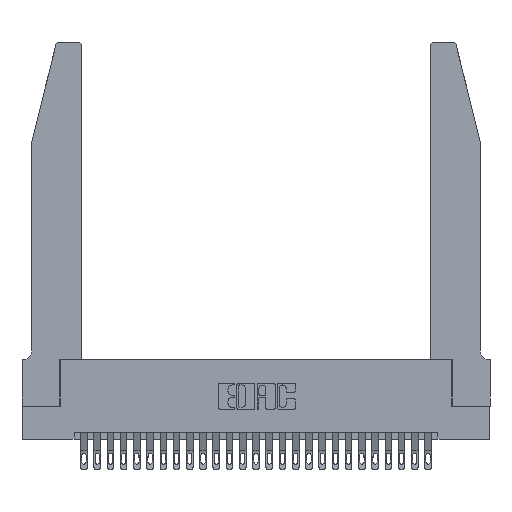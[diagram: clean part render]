
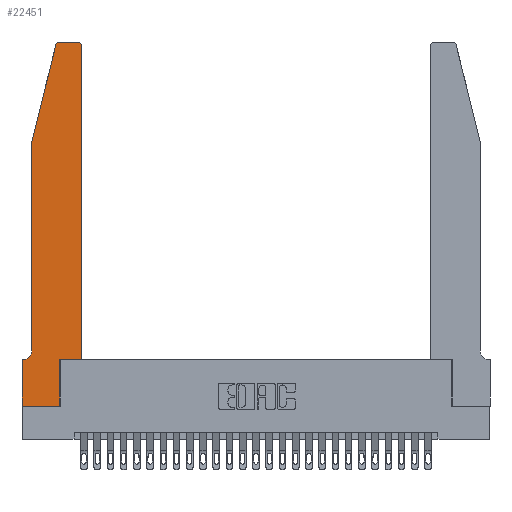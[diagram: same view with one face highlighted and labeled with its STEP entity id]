
A CAD part, top view. The second image highlights one B-rep face of the part: STEP entity #22451.
In plain terms, the highlighted planar face has unit normal (0, 0, 1).
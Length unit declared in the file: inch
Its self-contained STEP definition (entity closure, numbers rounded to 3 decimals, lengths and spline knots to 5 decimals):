
#262 = EDGE_CURVE ( 'NONE', #15563, #14935, #7388, .T. ) ;
#499 = LINE ( 'NONE', #13798, #14533 ) ;
#689 = DIRECTION ( 'NONE',  ( 0., -1., 0. ) ) ;
#719 = ORIENTED_EDGE ( 'NONE', *, *, #3942, .T. ) ;
#2291 = CARTESIAN_POINT ( 'NONE',  ( 0.2865, 0., 0.37 ) ) ;
#2309 = VERTEX_POINT ( 'NONE', #17809 ) ;
#2322 = CARTESIAN_POINT ( 'NONE',  ( 0.4505, 0.35, 0.37 ) ) ;
#2767 = VERTEX_POINT ( 'NONE', #3917 ) ;
#2889 = EDGE_CURVE ( 'NONE', #2767, #9014, #16793, .T. ) ;
#3114 = CARTESIAN_POINT ( 'NONE',  ( 0., 0.35, 0.37 ) ) ;
#3159 = CARTESIAN_POINT ( 'NONE',  ( 0.284, 2.72, 0.37 ) ) ;
#3435 = LINE ( 'NONE', #2322, #24571 ) ;
#3587 = VERTEX_POINT ( 'NONE', #7148 ) ;
#3636 = ORIENTED_EDGE ( 'NONE', *, *, #262, .T. ) ;
#3851 = FACE_OUTER_BOUND ( 'NONE', #5052, .T. ) ;
#3917 = CARTESIAN_POINT ( 'NONE',  ( 0.284, 2.75, 0.37 ) ) ;
#3942 = EDGE_CURVE ( 'NONE', #14935, #12916, #12689, .T. ) ;
#4130 = ORIENTED_EDGE ( 'NONE', *, *, #2889, .T. ) ;
#4731 = CARTESIAN_POINT ( 'NONE',  ( 0., 0., 0.37 ) ) ;
#5052 = EDGE_LOOP ( 'NONE', ( #22995, #4130, #22758, #17055, #23504, #27004, #26074, #15351, #3636, #719, #7775, #24972 ) ) ;
#5385 = DIRECTION ( 'NONE',  ( -0.239, -0.971, 0. ) ) ;
#5567 = CARTESIAN_POINT ( 'NONE',  ( 0.0755, 2., 0.37 ) ) ;
#5806 = CARTESIAN_POINT ( 'NONE',  ( 0.2865, 0.35, 0.37 ) ) ;
#6083 = VECTOR ( 'NONE', #8655, 39.37008 ) ;
#6572 = CARTESIAN_POINT ( 'NONE',  ( 0., 0., 0.37 ) ) ;
#6671 = VERTEX_POINT ( 'NONE', #7712 ) ;
#7032 = VECTOR ( 'NONE', #5385, 39.37008 ) ;
#7148 = CARTESIAN_POINT ( 'NONE',  ( 0.0755, 0.42, 0.37 ) ) ;
#7388 = LINE ( 'NONE', #5806, #25094 ) ;
#7712 = CARTESIAN_POINT ( 'NONE',  ( 0.4505, 2.72, 0.37 ) ) ;
#7775 = ORIENTED_EDGE ( 'NONE', *, *, #24024, .T. ) ;
#7969 = VERTEX_POINT ( 'NONE', #22263 ) ;
#7994 = CARTESIAN_POINT ( 'NONE',  ( 0.4505, 0.35, 0.37 ) ) ;
#8459 = DIRECTION ( 'NONE',  ( 0., 0., 1. ) ) ;
#8655 = DIRECTION ( 'NONE',  ( 0., -1., 0. ) ) ;
#9014 = VERTEX_POINT ( 'NONE', #11746 ) ;
#9114 = LINE ( 'NONE', #5567, #7032 ) ;
#10120 = CIRCLE ( 'NONE', #13296, 0.03 ) ;
#10205 = DIRECTION ( 'NONE',  ( 1., 0., 0. ) ) ;
#10240 = LINE ( 'NONE', #26243, #6083 ) ;
#10771 = CARTESIAN_POINT ( 'NONE',  ( 0.4505, 0.35, 0.37 ) ) ;
#10926 = EDGE_CURVE ( 'NONE', #3587, #7969, #12141, .T. ) ;
#11746 = CARTESIAN_POINT ( 'NONE',  ( 0.25487, 2.72718, 0.37 ) ) ;
#12011 = VERTEX_POINT ( 'NONE', #17319 ) ;
#12141 = CIRCLE ( 'NONE', #12174, 0.07 ) ;
#12174 = AXIS2_PLACEMENT_3D ( 'NONE', #18781, #26338, #17679 ) ;
#12653 = CARTESIAN_POINT ( 'NONE',  ( 0.0755, 2., 0.37 ) ) ;
#12689 = LINE ( 'NONE', #7994, #13353 ) ;
#12778 = CARTESIAN_POINT ( 'NONE',  ( 0.2605, 2.75, 0.37 ) ) ;
#12916 = VERTEX_POINT ( 'NONE', #10771 ) ;
#12948 = EDGE_CURVE ( 'NONE', #6671, #2309, #10120, .T. ) ;
#12950 = EDGE_CURVE ( 'NONE', #2309, #2767, #18228, .T. ) ;
#12952 = LINE ( 'NONE', #6572, #15974 ) ;
#13057 = CARTESIAN_POINT ( 'NONE',  ( 0.4205, 2.72, 0.37 ) ) ;
#13296 = AXIS2_PLACEMENT_3D ( 'NONE', #13057, #8459, #23609 ) ;
#13353 = VECTOR ( 'NONE', #10205, 39.37008 ) ;
#13798 = CARTESIAN_POINT ( 'NONE',  ( 0., 0., 0.37 ) ) ;
#14113 = DIRECTION ( 'NONE',  ( 1., 0., 0. ) ) ;
#14509 = DIRECTION ( 'NONE',  ( 0., 1., 0. ) ) ;
#14533 = VECTOR ( 'NONE', #689, 39.37008 ) ;
#14935 = VERTEX_POINT ( 'NONE', #23208 ) ;
#15153 = DIRECTION ( 'NONE',  ( -1., 0., 0. ) ) ;
#15351 = ORIENTED_EDGE ( 'NONE', *, *, #16845, .T. ) ;
#15563 = VERTEX_POINT ( 'NONE', #2291 ) ;
#15974 = VECTOR ( 'NONE', #23259, 39.37008 ) ;
#16793 = CIRCLE ( 'NONE', #26216, 0.03 ) ;
#16845 = EDGE_CURVE ( 'NONE', #19256, #15563, #12952, .T. ) ;
#16880 = EDGE_CURVE ( 'NONE', #7969, #12011, #28265, .T. ) ;
#17055 = ORIENTED_EDGE ( 'NONE', *, *, #25073, .T. ) ;
#17319 = CARTESIAN_POINT ( 'NONE',  ( 0., 0.35, 0.37 ) ) ;
#17679 = DIRECTION ( 'NONE',  ( -1., 0., 0. ) ) ;
#17809 = CARTESIAN_POINT ( 'NONE',  ( 0.4205, 2.75, 0.37 ) ) ;
#18004 = VECTOR ( 'NONE', #19179, 39.37008 ) ;
#18228 = LINE ( 'NONE', #12778, #19900 ) ;
#18397 = DIRECTION ( 'NONE',  ( 0., 0., 1. ) ) ;
#18777 = PLANE ( 'NONE',  #28030 ) ;
#18781 = CARTESIAN_POINT ( 'NONE',  ( 0.0055, 0.42, 0.37 ) ) ;
#19179 = DIRECTION ( 'NONE',  ( -1., 0., 0. ) ) ;
#19256 = VERTEX_POINT ( 'NONE', #4731 ) ;
#19900 = VECTOR ( 'NONE', #15153, 39.37008 ) ;
#20604 = DIRECTION ( 'NONE',  ( 0., 0., 1. ) ) ;
#20747 = EDGE_CURVE ( 'NONE', #9014, #24419, #9114, .T. ) ;
#22263 = CARTESIAN_POINT ( 'NONE',  ( 0.0055, 0.35, 0.37 ) ) ;
#22451 = ADVANCED_FACE ( 'NONE', ( #3851 ), #18777, .T. ) ;
#22758 = ORIENTED_EDGE ( 'NONE', *, *, #20747, .T. ) ;
#22995 = ORIENTED_EDGE ( 'NONE', *, *, #12950, .T. ) ;
#23208 = CARTESIAN_POINT ( 'NONE',  ( 0.2865, 0.35, 0.37 ) ) ;
#23259 = DIRECTION ( 'NONE',  ( 1., 0., 0. ) ) ;
#23471 = DIRECTION ( 'NONE',  ( 1., 0., 0. ) ) ;
#23504 = ORIENTED_EDGE ( 'NONE', *, *, #10926, .T. ) ;
#23609 = DIRECTION ( 'NONE',  ( 1., 0., 0. ) ) ;
#24024 = EDGE_CURVE ( 'NONE', #12916, #6671, #3435, .T. ) ;
#24419 = VERTEX_POINT ( 'NONE', #12653 ) ;
#24571 = VECTOR ( 'NONE', #26828, 39.37008 ) ;
#24972 = ORIENTED_EDGE ( 'NONE', *, *, #12948, .T. ) ;
#25073 = EDGE_CURVE ( 'NONE', #24419, #3587, #10240, .T. ) ;
#25094 = VECTOR ( 'NONE', #14509, 39.37008 ) ;
#25726 = CARTESIAN_POINT ( 'NONE',  ( 0.0755, 0.35, 0.37 ) ) ;
#26074 = ORIENTED_EDGE ( 'NONE', *, *, #27007, .T. ) ;
#26216 = AXIS2_PLACEMENT_3D ( 'NONE', #3159, #20604, #23471 ) ;
#26243 = CARTESIAN_POINT ( 'NONE',  ( 0.0755, 2., 0.37 ) ) ;
#26338 = DIRECTION ( 'NONE',  ( 0., 0., -1. ) ) ;
#26828 = DIRECTION ( 'NONE',  ( 0., 1., 0. ) ) ;
#27004 = ORIENTED_EDGE ( 'NONE', *, *, #16880, .T. ) ;
#27007 = EDGE_CURVE ( 'NONE', #12011, #19256, #499, .T. ) ;
#28030 = AXIS2_PLACEMENT_3D ( 'NONE', #3114, #18397, #14113 ) ;
#28265 = LINE ( 'NONE', #25726, #18004 ) ;
